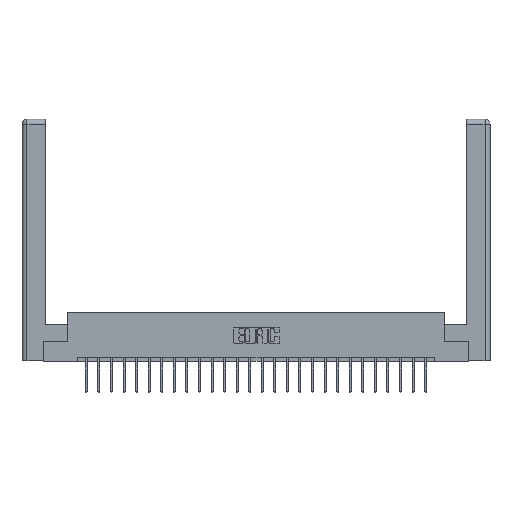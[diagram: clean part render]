
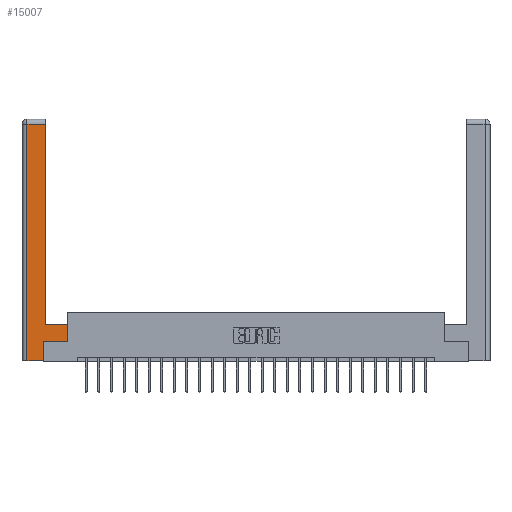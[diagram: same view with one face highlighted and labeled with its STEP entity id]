
A CAD part, top view. The second image highlights one B-rep face of the part: STEP entity #15007.
In plain terms, the highlighted planar face has unit normal (0, 0, 1).
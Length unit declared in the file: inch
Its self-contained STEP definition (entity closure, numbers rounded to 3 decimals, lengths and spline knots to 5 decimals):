
#107 = CARTESIAN_POINT ( 'NONE',  ( 0.295, 3., 0. ) ) ;
#394 = EDGE_CURVE ( 'NONE', #19321, #24374, #14945, .T. ) ;
#1159 = AXIS2_PLACEMENT_3D ( 'NONE', #2312, #8438, #8614 ) ;
#1190 = DIRECTION ( 'NONE',  ( -1., 0., 0. ) ) ;
#1330 = LINE ( 'NONE', #107, #22222 ) ;
#1814 = CARTESIAN_POINT ( 'NONE',  ( 0.0615, 0., 0. ) ) ;
#2312 = CARTESIAN_POINT ( 'NONE',  ( 0., 0., 0. ) ) ;
#2905 = ORIENTED_EDGE ( 'NONE', *, *, #23463, .T. ) ;
#3581 = DIRECTION ( 'NONE',  ( 0., 1., 0. ) ) ;
#4224 = VECTOR ( 'NONE', #12429, 39.37008 ) ;
#4337 = VECTOR ( 'NONE', #7280, 39.37008 ) ;
#4612 = ORIENTED_EDGE ( 'NONE', *, *, #25971, .T. ) ;
#4681 = CARTESIAN_POINT ( 'NONE',  ( 0.265, 0., 0. ) ) ;
#4683 = VERTEX_POINT ( 'NONE', #10651 ) ;
#5466 = VERTEX_POINT ( 'NONE', #5645 ) ;
#5645 = CARTESIAN_POINT ( 'NONE',  ( 0.565, 0.45, 0. ) ) ;
#5749 = EDGE_CURVE ( 'NONE', #17786, #6957, #23190, .T. ) ;
#5767 = CARTESIAN_POINT ( 'NONE',  ( 0.565, 0.45, 0. ) ) ;
#6324 = CARTESIAN_POINT ( 'NONE',  ( 0.265, 0., 0. ) ) ;
#6896 = ORIENTED_EDGE ( 'NONE', *, *, #15313, .T. ) ;
#6957 = VERTEX_POINT ( 'NONE', #23064 ) ;
#7280 = DIRECTION ( 'NONE',  ( 0., -1., 0. ) ) ;
#7451 = DIRECTION ( 'NONE',  ( 1., 0., 0. ) ) ;
#7668 = CARTESIAN_POINT ( 'NONE',  ( 0.265, 0.245, 0. ) ) ;
#8438 = DIRECTION ( 'NONE',  ( 0., 0., -1. ) ) ;
#8506 = LINE ( 'NONE', #12976, #22592 ) ;
#8614 = DIRECTION ( 'NONE',  ( -1., 0., 0. ) ) ;
#8902 = EDGE_CURVE ( 'NONE', #4683, #5466, #12599, .T. ) ;
#9520 = VECTOR ( 'NONE', #11484, 39.37008 ) ;
#10297 = EDGE_LOOP ( 'NONE', ( #24842, #14751, #15703, #16278, #4612, #6896, #16037, #2905 ) ) ;
#10443 = PLANE ( 'NONE',  #1159 ) ;
#10651 = CARTESIAN_POINT ( 'NONE',  ( 0.565, 0.245, 0. ) ) ;
#10908 = DIRECTION ( 'NONE',  ( -1., 0., 0. ) ) ;
#10991 = VECTOR ( 'NONE', #3581, 39.37008 ) ;
#11484 = DIRECTION ( 'NONE',  ( 0., 1., 0. ) ) ;
#12429 = DIRECTION ( 'NONE',  ( 1., 0., 0. ) ) ;
#12599 = LINE ( 'NONE', #5767, #10991 ) ;
#12976 = CARTESIAN_POINT ( 'NONE',  ( 0.295, 0.45, 0. ) ) ;
#13074 = VECTOR ( 'NONE', #10908, 39.37008 ) ;
#13114 = EDGE_CURVE ( 'NONE', #6957, #19321, #19521, .T. ) ;
#13198 = CARTESIAN_POINT ( 'NONE',  ( 0.0615, 0., 0. ) ) ;
#14751 = ORIENTED_EDGE ( 'NONE', *, *, #5749, .T. ) ;
#14870 = LINE ( 'NONE', #21493, #9520 ) ;
#14943 = CARTESIAN_POINT ( 'NONE',  ( 0.295, 0.45, 0. ) ) ;
#14945 = LINE ( 'NONE', #6324, #4224 ) ;
#15001 = EDGE_CURVE ( 'NONE', #21531, #17786, #1330, .T. ) ;
#15007 = ADVANCED_FACE ( 'NONE', ( #20983 ), #10443, .F. ) ;
#15313 = EDGE_CURVE ( 'NONE', #24698, #4683, #15904, .T. ) ;
#15703 = ORIENTED_EDGE ( 'NONE', *, *, #13114, .T. ) ;
#15904 = LINE ( 'NONE', #25298, #17172 ) ;
#16037 = ORIENTED_EDGE ( 'NONE', *, *, #8902, .T. ) ;
#16278 = ORIENTED_EDGE ( 'NONE', *, *, #394, .T. ) ;
#17083 = CARTESIAN_POINT ( 'NONE',  ( 0.0615, 2.94, 0. ) ) ;
#17172 = VECTOR ( 'NONE', #7451, 39.37008 ) ;
#17786 = VERTEX_POINT ( 'NONE', #24904 ) ;
#18415 = DIRECTION ( 'NONE',  ( 0., 1., 0. ) ) ;
#19321 = VERTEX_POINT ( 'NONE', #1814 ) ;
#19521 = LINE ( 'NONE', #13198, #4337 ) ;
#20983 = FACE_OUTER_BOUND ( 'NONE', #10297, .T. ) ;
#21493 = CARTESIAN_POINT ( 'NONE',  ( 0.265, 0.245, 0. ) ) ;
#21531 = VERTEX_POINT ( 'NONE', #14943 ) ;
#22222 = VECTOR ( 'NONE', #18415, 39.37008 ) ;
#22592 = VECTOR ( 'NONE', #1190, 39.37008 ) ;
#23064 = CARTESIAN_POINT ( 'NONE',  ( 0.0615, 2.94, 0. ) ) ;
#23190 = LINE ( 'NONE', #17083, #13074 ) ;
#23463 = EDGE_CURVE ( 'NONE', #5466, #21531, #8506, .T. ) ;
#24374 = VERTEX_POINT ( 'NONE', #4681 ) ;
#24698 = VERTEX_POINT ( 'NONE', #7668 ) ;
#24842 = ORIENTED_EDGE ( 'NONE', *, *, #15001, .T. ) ;
#24904 = CARTESIAN_POINT ( 'NONE',  ( 0.295, 2.94, 0. ) ) ;
#25298 = CARTESIAN_POINT ( 'NONE',  ( 0.565, 0.245, 0. ) ) ;
#25971 = EDGE_CURVE ( 'NONE', #24374, #24698, #14870, .T. ) ;
